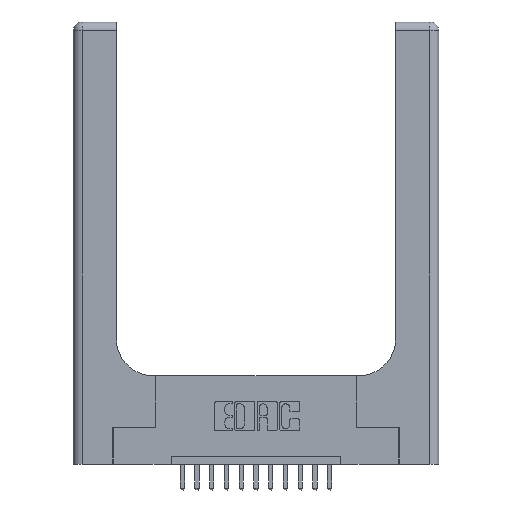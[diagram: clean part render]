
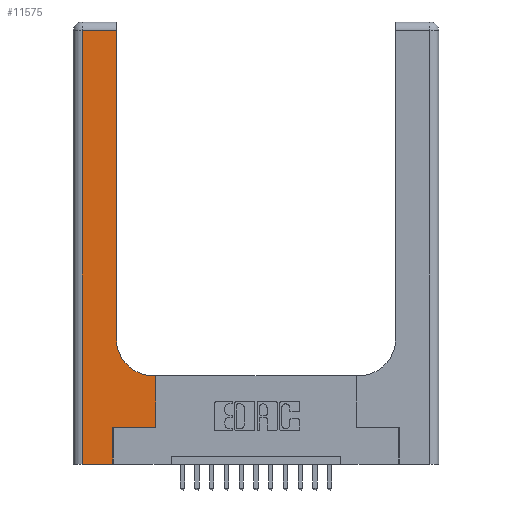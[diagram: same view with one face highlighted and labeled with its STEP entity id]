
A CAD part, top view. The second image highlights one B-rep face of the part: STEP entity #11575.
In plain terms, the highlighted planar face has unit normal (0, 0, 1).
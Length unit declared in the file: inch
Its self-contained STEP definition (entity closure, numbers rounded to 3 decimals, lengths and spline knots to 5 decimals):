
#214 = CARTESIAN_POINT ( 'NONE',  ( 0.2915, 0.6, 0.37 ) ) ;
#519 = EDGE_CURVE ( 'NONE', #3624, #761, #9760, .T. ) ;
#536 = LINE ( 'NONE', #3004, #4026 ) ;
#555 = VERTEX_POINT ( 'NONE', #11254 ) ;
#582 = CARTESIAN_POINT ( 'NONE',  ( 0.269, 0., 0.37 ) ) ;
#761 = VERTEX_POINT ( 'NONE', #17131 ) ;
#1004 = DIRECTION ( 'NONE',  ( 0., 0., -1. ) ) ;
#1350 = PLANE ( 'NONE',  #12793 ) ;
#1549 = EDGE_CURVE ( 'NONE', #5555, #16254, #7811, .T. ) ;
#1574 = EDGE_CURVE ( 'NONE', #555, #15883, #9931, .T. ) ;
#2223 = ORIENTED_EDGE ( 'NONE', *, *, #519, .T. ) ;
#2470 = DIRECTION ( 'NONE',  ( 1., 0., 0. ) ) ;
#3004 = CARTESIAN_POINT ( 'NONE',  ( 0.06, 3., 0.37 ) ) ;
#3343 = DIRECTION ( 'NONE',  ( -1., 0., 0. ) ) ;
#3624 = VERTEX_POINT ( 'NONE', #5990 ) ;
#3678 = ORIENTED_EDGE ( 'NONE', *, *, #10717, .T. ) ;
#3822 = CARTESIAN_POINT ( 'NONE',  ( 0.269, 0., 0.37 ) ) ;
#3981 = ORIENTED_EDGE ( 'NONE', *, *, #10896, .T. ) ;
#4026 = VECTOR ( 'NONE', #8633, 39.37008 ) ;
#5128 = ORIENTED_EDGE ( 'NONE', *, *, #1549, .T. ) ;
#5271 = VECTOR ( 'NONE', #7302, 39.37008 ) ;
#5555 = VERTEX_POINT ( 'NONE', #14505 ) ;
#5990 = CARTESIAN_POINT ( 'NONE',  ( 0.5585, 0.6, 0.37 ) ) ;
#6584 = DIRECTION ( 'NONE',  ( 0., 1., 0. ) ) ;
#6628 = LINE ( 'NONE', #11244, #14578 ) ;
#6916 = DIRECTION ( 'NONE',  ( 1., 0., 0. ) ) ;
#6955 = ORIENTED_EDGE ( 'NONE', *, *, #1574, .T. ) ;
#6996 = CARTESIAN_POINT ( 'NONE',  ( 0., 3., 0.37 ) ) ;
#7302 = DIRECTION ( 'NONE',  ( -1., 0., 0. ) ) ;
#7365 = VERTEX_POINT ( 'NONE', #13346 ) ;
#7385 = ORIENTED_EDGE ( 'NONE', *, *, #13869, .T. ) ;
#7598 = VECTOR ( 'NONE', #14744, 39.37008 ) ;
#7811 = LINE ( 'NONE', #14802, #7598 ) ;
#7936 = CIRCLE ( 'NONE', #8268, 0.25 ) ;
#8268 = AXIS2_PLACEMENT_3D ( 'NONE', #17426, #1004, #2470 ) ;
#8436 = CARTESIAN_POINT ( 'NONE',  ( 0.5585, 0.25, 0.37 ) ) ;
#8457 = EDGE_CURVE ( 'NONE', #7365, #16135, #6628, .T. ) ;
#8633 = DIRECTION ( 'NONE',  ( 0., -1., 0. ) ) ;
#8640 = LINE ( 'NONE', #11302, #15089 ) ;
#9060 = ORIENTED_EDGE ( 'NONE', *, *, #8457, .T. ) ;
#9100 = CARTESIAN_POINT ( 'NONE',  ( 0.5585, 0.25, 0.37 ) ) ;
#9378 = VECTOR ( 'NONE', #15579, 39.37008 ) ;
#9760 = LINE ( 'NONE', #214, #5271 ) ;
#9931 = LINE ( 'NONE', #13749, #14904 ) ;
#10230 = DIRECTION ( 'NONE',  ( 0., 0., -1. ) ) ;
#10717 = EDGE_CURVE ( 'NONE', #15883, #3624, #11870, .T. ) ;
#10896 = EDGE_CURVE ( 'NONE', #16135, #14099, #8640, .T. ) ;
#11003 = VECTOR ( 'NONE', #13222, 39.37008 ) ;
#11060 = CARTESIAN_POINT ( 'NONE',  ( 0.06, 2.94, 0.37 ) ) ;
#11244 = CARTESIAN_POINT ( 'NONE',  ( 0.2915, 3., 0.37 ) ) ;
#11254 = CARTESIAN_POINT ( 'NONE',  ( 0.269, 0.25, 0.37 ) ) ;
#11302 = CARTESIAN_POINT ( 'NONE',  ( 0., 2.94, 0.37 ) ) ;
#11575 = ADVANCED_FACE ( 'NONE', ( #16555 ), #1350, .F. ) ;
#11870 = LINE ( 'NONE', #9100, #11003 ) ;
#12793 = AXIS2_PLACEMENT_3D ( 'NONE', #6996, #10230, #15714 ) ;
#12890 = CARTESIAN_POINT ( 'NONE',  ( 0.2915, 2.94, 0.37 ) ) ;
#13222 = DIRECTION ( 'NONE',  ( 0., 1., 0. ) ) ;
#13346 = CARTESIAN_POINT ( 'NONE',  ( 0.2915, 0.85, 0.37 ) ) ;
#13749 = CARTESIAN_POINT ( 'NONE',  ( 0.269, 0.25, 0.37 ) ) ;
#13869 = EDGE_CURVE ( 'NONE', #761, #7365, #7936, .T. ) ;
#14099 = VERTEX_POINT ( 'NONE', #11060 ) ;
#14500 = EDGE_LOOP ( 'NONE', ( #9060, #3981, #14797, #5128, #17677, #6955, #3678, #2223, #7385 ) ) ;
#14505 = CARTESIAN_POINT ( 'NONE',  ( 0.06, 0., 0.37 ) ) ;
#14578 = VECTOR ( 'NONE', #6584, 39.37008 ) ;
#14744 = DIRECTION ( 'NONE',  ( 1., 0., 0. ) ) ;
#14797 = ORIENTED_EDGE ( 'NONE', *, *, #14840, .T. ) ;
#14802 = CARTESIAN_POINT ( 'NONE',  ( 0., 0., 0.37 ) ) ;
#14840 = EDGE_CURVE ( 'NONE', #14099, #5555, #536, .T. ) ;
#14904 = VECTOR ( 'NONE', #6916, 39.37008 ) ;
#14933 = EDGE_CURVE ( 'NONE', #16254, #555, #16658, .T. ) ;
#15089 = VECTOR ( 'NONE', #3343, 39.37008 ) ;
#15579 = DIRECTION ( 'NONE',  ( 0., 1., 0. ) ) ;
#15714 = DIRECTION ( 'NONE',  ( -1., 0., 0. ) ) ;
#15883 = VERTEX_POINT ( 'NONE', #8436 ) ;
#16135 = VERTEX_POINT ( 'NONE', #12890 ) ;
#16254 = VERTEX_POINT ( 'NONE', #3822 ) ;
#16555 = FACE_OUTER_BOUND ( 'NONE', #14500, .T. ) ;
#16658 = LINE ( 'NONE', #582, #9378 ) ;
#17131 = CARTESIAN_POINT ( 'NONE',  ( 0.5415, 0.6, 0.37 ) ) ;
#17426 = CARTESIAN_POINT ( 'NONE',  ( 0.5415, 0.85, 0.37 ) ) ;
#17677 = ORIENTED_EDGE ( 'NONE', *, *, #14933, .T. ) ;
